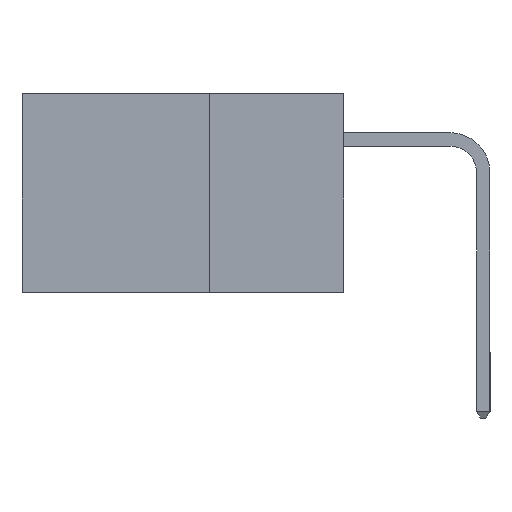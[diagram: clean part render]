
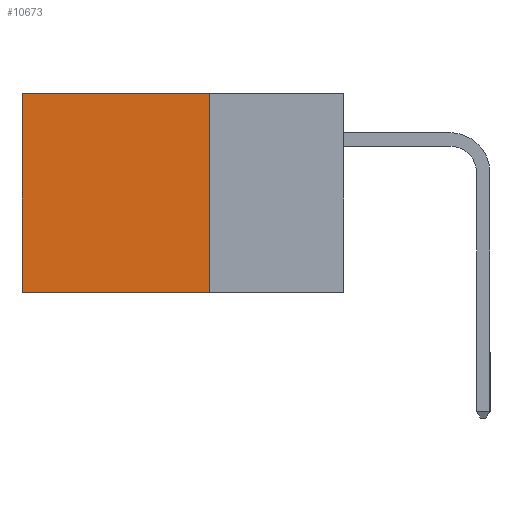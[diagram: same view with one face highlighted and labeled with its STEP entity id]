
A CAD part, left-side view. The second image highlights one B-rep face of the part: STEP entity #10673.
In plain terms, the highlighted planar face has unit normal (-1, 0, 0).
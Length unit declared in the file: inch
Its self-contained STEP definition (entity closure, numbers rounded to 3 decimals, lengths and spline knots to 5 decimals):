
#858 = LINE ( 'NONE', #30055, #13838 ) ;
#2623 = DIRECTION ( 'NONE',  ( 0., 0., -1. ) ) ;
#4393 = ORIENTED_EDGE ( 'NONE', *, *, #28325, .T. ) ;
#4516 = CARTESIAN_POINT ( 'NONE',  ( 0.298, 0.6, -0.37 ) ) ;
#4921 = VERTEX_POINT ( 'NONE', #25067 ) ;
#4969 = VECTOR ( 'NONE', #6030, 39.37008 ) ;
#5874 = ORIENTED_EDGE ( 'NONE', *, *, #29348, .T. ) ;
#6030 = DIRECTION ( 'NONE',  ( 0., 0., -1. ) ) ;
#6888 = VECTOR ( 'NONE', #14159, 39.37008 ) ;
#7032 = EDGE_CURVE ( 'NONE', #4921, #25827, #25594, .T. ) ;
#7474 = CARTESIAN_POINT ( 'NONE',  ( 0.298, 0.6, 0. ) ) ;
#9242 = EDGE_LOOP ( 'NONE', ( #4393, #29090, #10614, #5874 ) ) ;
#9312 = CARTESIAN_POINT ( 'NONE',  ( 0.298, 0.25, -0.37 ) ) ;
#10614 = ORIENTED_EDGE ( 'NONE', *, *, #21891, .F. ) ;
#10673 = ADVANCED_FACE ( 'NONE', ( #11216 ), #21536, .F. ) ;
#11216 = FACE_OUTER_BOUND ( 'NONE', #9242, .T. ) ;
#12264 = DIRECTION ( 'NONE',  ( 1., 0., 0. ) ) ;
#13838 = VECTOR ( 'NONE', #13944, 39.37008 ) ;
#13944 = DIRECTION ( 'NONE',  ( 0., 1., 0. ) ) ;
#14159 = DIRECTION ( 'NONE',  ( 0., 1., 0. ) ) ;
#15281 = AXIS2_PLACEMENT_3D ( 'NONE', #26126, #12264, #28416 ) ;
#17549 = VERTEX_POINT ( 'NONE', #18123 ) ;
#18123 = CARTESIAN_POINT ( 'NONE',  ( 0.298, 0.25, 0. ) ) ;
#21536 = PLANE ( 'NONE',  #15281 ) ;
#21891 = EDGE_CURVE ( 'NONE', #17549, #4921, #23843, .T. ) ;
#22088 = CARTESIAN_POINT ( 'NONE',  ( 0.298, 0.6, 0. ) ) ;
#22559 = CARTESIAN_POINT ( 'NONE',  ( 0.298, 0.25, 0. ) ) ;
#23843 = LINE ( 'NONE', #22559, #4969 ) ;
#25067 = CARTESIAN_POINT ( 'NONE',  ( 0.298, 0.25, -0.37 ) ) ;
#25078 = VECTOR ( 'NONE', #2623, 39.37008 ) ;
#25594 = LINE ( 'NONE', #9312, #6888 ) ;
#25827 = VERTEX_POINT ( 'NONE', #4516 ) ;
#26126 = CARTESIAN_POINT ( 'NONE',  ( 0.298, 0.25, 0. ) ) ;
#26514 = LINE ( 'NONE', #7474, #25078 ) ;
#28325 = EDGE_CURVE ( 'NONE', #30420, #25827, #26514, .T. ) ;
#28416 = DIRECTION ( 'NONE',  ( 0., 0., -1. ) ) ;
#29090 = ORIENTED_EDGE ( 'NONE', *, *, #7032, .F. ) ;
#29348 = EDGE_CURVE ( 'NONE', #17549, #30420, #858, .T. ) ;
#30055 = CARTESIAN_POINT ( 'NONE',  ( 0.298, 0.25, 0. ) ) ;
#30420 = VERTEX_POINT ( 'NONE', #22088 ) ;
